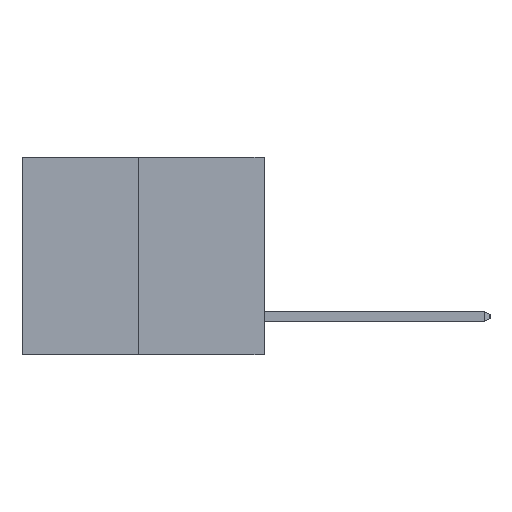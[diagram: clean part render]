
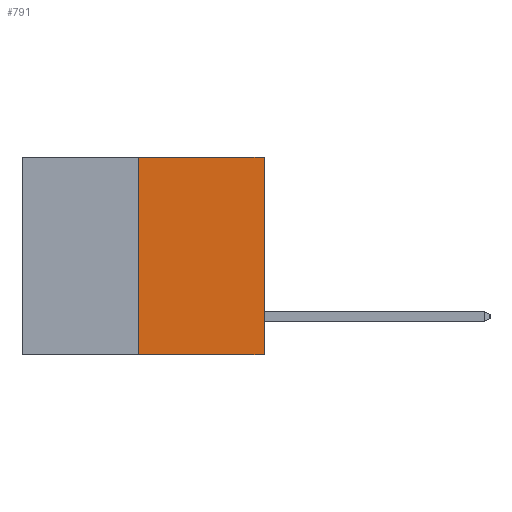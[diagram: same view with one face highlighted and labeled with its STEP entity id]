
A CAD part, left-side view. The second image highlights one B-rep face of the part: STEP entity #791.
In plain terms, the highlighted planar face has unit normal (-1, 0, 0).
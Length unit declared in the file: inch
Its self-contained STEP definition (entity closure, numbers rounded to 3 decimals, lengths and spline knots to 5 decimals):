
#642 = CARTESIAN_POINT ( 'NONE',  ( 0., 0.6, 0. ) ) ;
#791 = ADVANCED_FACE ( 'NONE', ( #3677 ), #9257, .F. ) ;
#2063 = DIRECTION ( 'NONE',  ( 0., 0., -1. ) ) ;
#2071 = CARTESIAN_POINT ( 'NONE',  ( 0., 0.6, -0.49 ) ) ;
#2767 = DIRECTION ( 'NONE',  ( 0., 0., 1. ) ) ;
#3296 = LINE ( 'NONE', #5513, #18584 ) ;
#3472 = ORIENTED_EDGE ( 'NONE', *, *, #18585, .F. ) ;
#3677 = FACE_OUTER_BOUND ( 'NONE', #12693, .T. ) ;
#5003 = DIRECTION ( 'NONE',  ( 0., 0., 1. ) ) ;
#5461 = EDGE_CURVE ( 'NONE', #6324, #5541, #8481, .T. ) ;
#5513 = CARTESIAN_POINT ( 'NONE',  ( 0., 0.6, 0. ) ) ;
#5541 = VERTEX_POINT ( 'NONE', #16997 ) ;
#6324 = VERTEX_POINT ( 'NONE', #12523 ) ;
#6352 = DIRECTION ( 'NONE',  ( 1., 0., 0. ) ) ;
#6534 = LINE ( 'NONE', #2071, #11435 ) ;
#6932 = DIRECTION ( 'NONE',  ( 0., -1., 0. ) ) ;
#7427 = CARTESIAN_POINT ( 'NONE',  ( 0., 0.312, -0.49 ) ) ;
#7661 = LINE ( 'NONE', #7427, #17873 ) ;
#8481 = LINE ( 'NONE', #13814, #14986 ) ;
#9257 = PLANE ( 'NONE',  #12042 ) ;
#10253 = ORIENTED_EDGE ( 'NONE', *, *, #15150, .T. ) ;
#11026 = DIRECTION ( 'NONE',  ( 0., -1., 0. ) ) ;
#11368 = VERTEX_POINT ( 'NONE', #11669 ) ;
#11435 = VECTOR ( 'NONE', #11026, 39.37008 ) ;
#11630 = ORIENTED_EDGE ( 'NONE', *, *, #5461, .T. ) ;
#11669 = CARTESIAN_POINT ( 'NONE',  ( 0., 0.312, -0.49 ) ) ;
#12042 = AXIS2_PLACEMENT_3D ( 'NONE', #642, #6352, #2063 ) ;
#12523 = CARTESIAN_POINT ( 'NONE',  ( 0., 0., -0.49 ) ) ;
#12693 = EDGE_LOOP ( 'NONE', ( #3472, #10253, #11630, #17868 ) ) ;
#13483 = CARTESIAN_POINT ( 'NONE',  ( 0., 0.312, 0. ) ) ;
#13814 = CARTESIAN_POINT ( 'NONE',  ( 0., 0., 0. ) ) ;
#14986 = VECTOR ( 'NONE', #5003, 39.37008 ) ;
#15150 = EDGE_CURVE ( 'NONE', #11368, #6324, #6534, .T. ) ;
#15244 = EDGE_CURVE ( 'NONE', #18087, #5541, #3296, .T. ) ;
#16997 = CARTESIAN_POINT ( 'NONE',  ( 0., 0., 0. ) ) ;
#17868 = ORIENTED_EDGE ( 'NONE', *, *, #15244, .F. ) ;
#17873 = VECTOR ( 'NONE', #2767, 39.37008 ) ;
#18087 = VERTEX_POINT ( 'NONE', #13483 ) ;
#18584 = VECTOR ( 'NONE', #6932, 39.37008 ) ;
#18585 = EDGE_CURVE ( 'NONE', #11368, #18087, #7661, .T. ) ;
